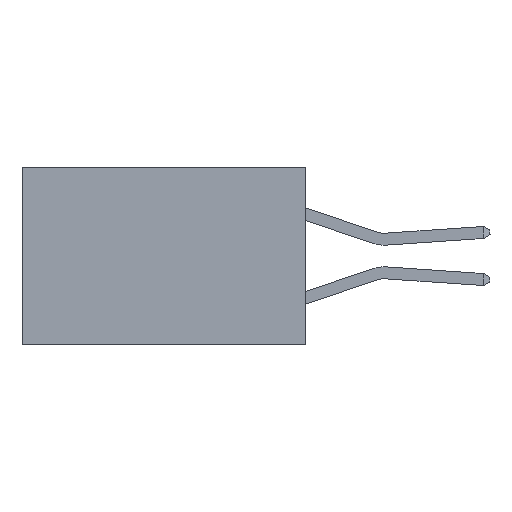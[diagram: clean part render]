
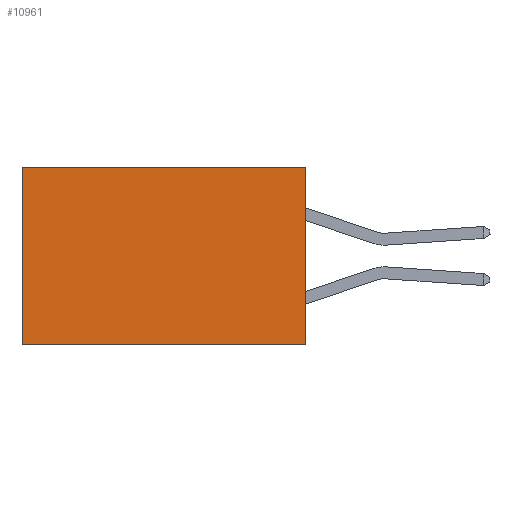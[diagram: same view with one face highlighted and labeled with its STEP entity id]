
A CAD part, left-side view. The second image highlights one B-rep face of the part: STEP entity #10961.
In plain terms, the highlighted planar face has unit normal (-1, 0, 0).
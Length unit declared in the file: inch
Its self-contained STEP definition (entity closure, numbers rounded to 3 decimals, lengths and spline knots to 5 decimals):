
#337 = CARTESIAN_POINT ( 'NONE',  ( 0.277, 0., -0.37 ) ) ;
#1304 = EDGE_CURVE ( 'NONE', #7650, #13063, #15561, .T. ) ;
#1803 = LINE ( 'NONE', #14486, #12827 ) ;
#2016 = ORIENTED_EDGE ( 'NONE', *, *, #1304, .T. ) ;
#2106 = CARTESIAN_POINT ( 'NONE',  ( 0.277, 0., 0. ) ) ;
#2128 = EDGE_CURVE ( 'NONE', #7650, #7943, #6331, .T. ) ;
#2502 = AXIS2_PLACEMENT_3D ( 'NONE', #5503, #12316, #4320 ) ;
#2721 = CARTESIAN_POINT ( 'NONE',  ( 0.277, 0., -0.37 ) ) ;
#4320 = DIRECTION ( 'NONE',  ( 0., 0., -1. ) ) ;
#5060 = EDGE_LOOP ( 'NONE', ( #9716, #13626, #15213, #2016 ) ) ;
#5503 = CARTESIAN_POINT ( 'NONE',  ( 0.277, 0., -0.37 ) ) ;
#6331 = LINE ( 'NONE', #2721, #12978 ) ;
#6599 = DIRECTION ( 'NONE',  ( 0., 0., -1. ) ) ;
#7650 = VERTEX_POINT ( 'NONE', #2106 ) ;
#7943 = VERTEX_POINT ( 'NONE', #337 ) ;
#7967 = CARTESIAN_POINT ( 'NONE',  ( 0.277, 0., 0. ) ) ;
#9070 = VECTOR ( 'NONE', #11661, 39.37008 ) ;
#9472 = CARTESIAN_POINT ( 'NONE',  ( 0.277, 0., -0.37 ) ) ;
#9716 = ORIENTED_EDGE ( 'NONE', *, *, #13979, .T. ) ;
#10961 = ADVANCED_FACE ( 'NONE', ( #16079 ), #10997, .F. ) ;
#10997 = PLANE ( 'NONE',  #2502 ) ;
#11661 = DIRECTION ( 'NONE',  ( 0., 1., 0. ) ) ;
#12316 = DIRECTION ( 'NONE',  ( 1., 0., 0. ) ) ;
#12331 = DIRECTION ( 'NONE',  ( 0., 0., -1. ) ) ;
#12595 = VERTEX_POINT ( 'NONE', #14292 ) ;
#12827 = VECTOR ( 'NONE', #6599, 39.37008 ) ;
#12978 = VECTOR ( 'NONE', #12331, 39.37008 ) ;
#13063 = VERTEX_POINT ( 'NONE', #13894 ) ;
#13626 = ORIENTED_EDGE ( 'NONE', *, *, #15437, .F. ) ;
#13787 = LINE ( 'NONE', #9472, #16683 ) ;
#13894 = CARTESIAN_POINT ( 'NONE',  ( 0.277, 0.59, 0. ) ) ;
#13979 = EDGE_CURVE ( 'NONE', #13063, #12595, #1803, .T. ) ;
#14292 = CARTESIAN_POINT ( 'NONE',  ( 0.277, 0.59, -0.37 ) ) ;
#14486 = CARTESIAN_POINT ( 'NONE',  ( 0.277, 0.59, -0.37 ) ) ;
#14719 = DIRECTION ( 'NONE',  ( 0., 1., 0. ) ) ;
#15213 = ORIENTED_EDGE ( 'NONE', *, *, #2128, .F. ) ;
#15437 = EDGE_CURVE ( 'NONE', #7943, #12595, #13787, .T. ) ;
#15561 = LINE ( 'NONE', #7967, #9070 ) ;
#16079 = FACE_OUTER_BOUND ( 'NONE', #5060, .T. ) ;
#16683 = VECTOR ( 'NONE', #14719, 39.37008 ) ;
